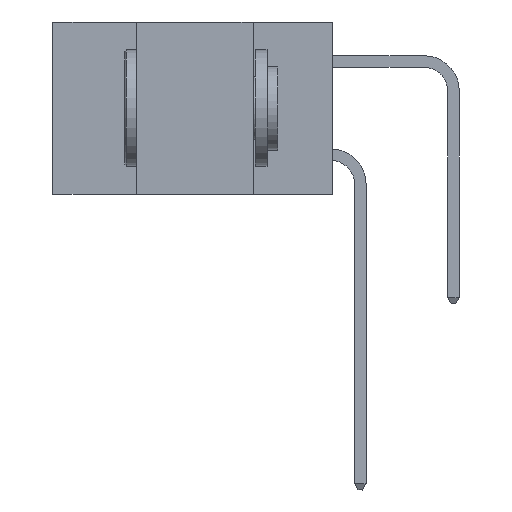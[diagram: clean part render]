
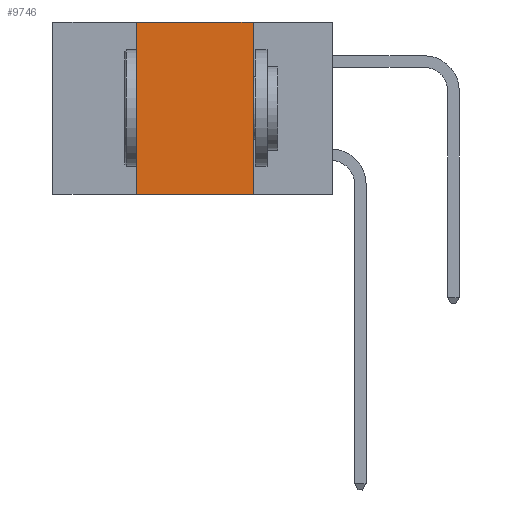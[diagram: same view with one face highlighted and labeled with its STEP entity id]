
A CAD part, left-side view. The second image highlights one B-rep face of the part: STEP entity #9746.
In plain terms, the highlighted planar face has unit normal (-1, 0, 0).
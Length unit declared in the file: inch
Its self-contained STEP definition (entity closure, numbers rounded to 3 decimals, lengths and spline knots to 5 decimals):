
#704 = CARTESIAN_POINT ( 'NONE',  ( 0., 0.42, -0.37 ) ) ;
#893 = CARTESIAN_POINT ( 'NONE',  ( 0., 0.17, 0. ) ) ;
#1684 = DIRECTION ( 'NONE',  ( 1., 0., 0. ) ) ;
#2430 = CARTESIAN_POINT ( 'NONE',  ( 0., 0.17, -0.37 ) ) ;
#2710 = LINE ( 'NONE', #10536, #7801 ) ;
#2778 = CARTESIAN_POINT ( 'NONE',  ( 0., 0.17, 0. ) ) ;
#4132 = LINE ( 'NONE', #6943, #6519 ) ;
#4468 = EDGE_CURVE ( 'NONE', #13006, #6337, #4132, .T. ) ;
#5117 = ORIENTED_EDGE ( 'NONE', *, *, #9810, .F. ) ;
#5154 = CARTESIAN_POINT ( 'NONE',  ( 0., 0.6, 0. ) ) ;
#5330 = CARTESIAN_POINT ( 'NONE',  ( 0., 0.42, 0. ) ) ;
#5722 = DIRECTION ( 'NONE',  ( 0., -1., 0. ) ) ;
#5857 = VECTOR ( 'NONE', #11477, 39.37008 ) ;
#6337 = VERTEX_POINT ( 'NONE', #2778 ) ;
#6519 = VECTOR ( 'NONE', #5722, 39.37008 ) ;
#6943 = CARTESIAN_POINT ( 'NONE',  ( 0., 0.6, 0. ) ) ;
#7291 = VERTEX_POINT ( 'NONE', #2430 ) ;
#7312 = ORIENTED_EDGE ( 'NONE', *, *, #4468, .F. ) ;
#7554 = PLANE ( 'NONE',  #14689 ) ;
#7801 = VECTOR ( 'NONE', #12791, 39.37008 ) ;
#7821 = CARTESIAN_POINT ( 'NONE',  ( 0., 0.42, 0. ) ) ;
#8805 = FACE_OUTER_BOUND ( 'NONE', #9028, .T. ) ;
#8848 = ORIENTED_EDGE ( 'NONE', *, *, #11423, .F. ) ;
#9028 = EDGE_LOOP ( 'NONE', ( #8848, #7312, #5117, #13924 ) ) ;
#9746 = ADVANCED_FACE ( 'NONE', ( #8805 ), #7554, .F. ) ;
#9809 = VERTEX_POINT ( 'NONE', #704 ) ;
#9810 = EDGE_CURVE ( 'NONE', #9809, #13006, #10086, .T. ) ;
#10071 = DIRECTION ( 'NONE',  ( 0., 0., 1. ) ) ;
#10086 = LINE ( 'NONE', #7821, #15030 ) ;
#10536 = CARTESIAN_POINT ( 'NONE',  ( 0., 0.6, -0.37 ) ) ;
#11401 = DIRECTION ( 'NONE',  ( 0., 0., -1. ) ) ;
#11423 = EDGE_CURVE ( 'NONE', #6337, #7291, #12554, .T. ) ;
#11477 = DIRECTION ( 'NONE',  ( 0., 0., -1. ) ) ;
#12554 = LINE ( 'NONE', #893, #5857 ) ;
#12660 = EDGE_CURVE ( 'NONE', #9809, #7291, #2710, .T. ) ;
#12791 = DIRECTION ( 'NONE',  ( 0., -1., 0. ) ) ;
#13006 = VERTEX_POINT ( 'NONE', #5330 ) ;
#13924 = ORIENTED_EDGE ( 'NONE', *, *, #12660, .T. ) ;
#14689 = AXIS2_PLACEMENT_3D ( 'NONE', #5154, #1684, #11401 ) ;
#15030 = VECTOR ( 'NONE', #10071, 39.37008 ) ;
